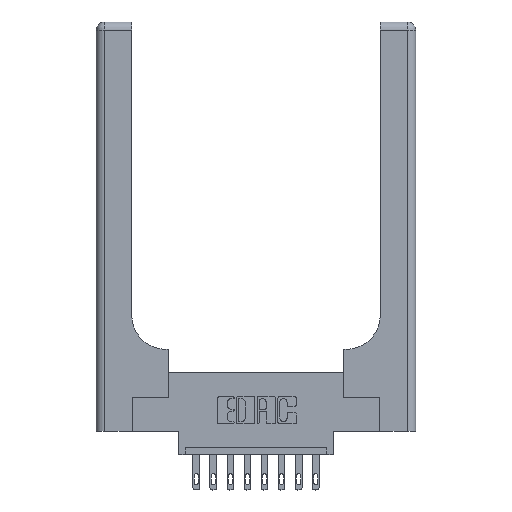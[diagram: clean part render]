
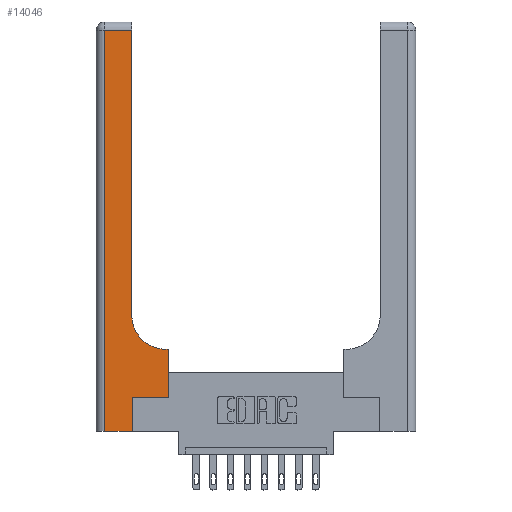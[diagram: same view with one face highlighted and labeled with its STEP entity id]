
A CAD part, top view. The second image highlights one B-rep face of the part: STEP entity #14046.
In plain terms, the highlighted planar face has unit normal (0, 0, 1).
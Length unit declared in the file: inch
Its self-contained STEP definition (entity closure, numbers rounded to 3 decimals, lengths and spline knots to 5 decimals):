
#158 = CARTESIAN_POINT ( 'NONE',  ( 0.265, 0., 0.37 ) ) ;
#459 = LINE ( 'NONE', #7547, #9441 ) ;
#603 = CARTESIAN_POINT ( 'NONE',  ( 0.26, 3., 0.37 ) ) ;
#756 = EDGE_LOOP ( 'NONE', ( #848, #13012, #11049, #14284, #3044, #6125, #1793, #9005, #6322 ) ) ;
#787 = CARTESIAN_POINT ( 'NONE',  ( 0.26, 2.94, 0.37 ) ) ;
#848 = ORIENTED_EDGE ( 'NONE', *, *, #12270, .T. ) ;
#910 = CARTESIAN_POINT ( 'NONE',  ( 0.26, 0.6, 0.37 ) ) ;
#918 = CARTESIAN_POINT ( 'NONE',  ( 0.528, 0.6, 0.37 ) ) ;
#1620 = LINE ( 'NONE', #603, #10219 ) ;
#1672 = DIRECTION ( 'NONE',  ( 0., -1., 0. ) ) ;
#1793 = ORIENTED_EDGE ( 'NONE', *, *, #2515, .T. ) ;
#2161 = VECTOR ( 'NONE', #14399, 39.37008 ) ;
#2469 = LINE ( 'NONE', #7157, #3348 ) ;
#2515 = EDGE_CURVE ( 'NONE', #13870, #5952, #8807, .T. ) ;
#3044 = ORIENTED_EDGE ( 'NONE', *, *, #3825, .T. ) ;
#3224 = CARTESIAN_POINT ( 'NONE',  ( 0.26, 0.85, 0.37 ) ) ;
#3348 = VECTOR ( 'NONE', #13458, 39.37008 ) ;
#3782 = VERTEX_POINT ( 'NONE', #4012 ) ;
#3825 = EDGE_CURVE ( 'NONE', #9197, #3782, #459, .T. ) ;
#3858 = DIRECTION ( 'NONE',  ( 0., 1., 0. ) ) ;
#4012 = CARTESIAN_POINT ( 'NONE',  ( 0.265, 0.25, 0.37 ) ) ;
#4062 = CARTESIAN_POINT ( 'NONE',  ( 0.06, 3., 0.37 ) ) ;
#4175 = CARTESIAN_POINT ( 'NONE',  ( 0.06, 2.94, 0.37 ) ) ;
#4379 = CARTESIAN_POINT ( 'NONE',  ( 0.51, 0.6, 0.37 ) ) ;
#4477 = DIRECTION ( 'NONE',  ( -1., 0., 0. ) ) ;
#4749 = VERTEX_POINT ( 'NONE', #4175 ) ;
#4796 = EDGE_CURVE ( 'NONE', #11384, #4749, #5330, .T. ) ;
#4879 = CARTESIAN_POINT ( 'NONE',  ( 0.265, 0.25, 0.37 ) ) ;
#5036 = LINE ( 'NONE', #4879, #2161 ) ;
#5330 = LINE ( 'NONE', #10004, #14877 ) ;
#5911 = CARTESIAN_POINT ( 'NONE',  ( 0.528, 0.25, 0.37 ) ) ;
#5952 = VERTEX_POINT ( 'NONE', #918 ) ;
#6125 = ORIENTED_EDGE ( 'NONE', *, *, #10378, .T. ) ;
#6128 = AXIS2_PLACEMENT_3D ( 'NONE', #6481, #12416, #11115 ) ;
#6322 = ORIENTED_EDGE ( 'NONE', *, *, #10534, .T. ) ;
#6481 = CARTESIAN_POINT ( 'NONE',  ( 0.51, 0.85, 0.37 ) ) ;
#6900 = VECTOR ( 'NONE', #1672, 39.37008 ) ;
#7157 = CARTESIAN_POINT ( 'NONE',  ( 0., 0., 0.37 ) ) ;
#7434 = CARTESIAN_POINT ( 'NONE',  ( 0., 3., 0.37 ) ) ;
#7547 = CARTESIAN_POINT ( 'NONE',  ( 0.265, 0., 0.37 ) ) ;
#7729 = VERTEX_POINT ( 'NONE', #4379 ) ;
#8346 = EDGE_CURVE ( 'NONE', #4749, #13665, #11228, .T. ) ;
#8807 = LINE ( 'NONE', #12158, #14511 ) ;
#9005 = ORIENTED_EDGE ( 'NONE', *, *, #12449, .T. ) ;
#9197 = VERTEX_POINT ( 'NONE', #158 ) ;
#9318 = VECTOR ( 'NONE', #4477, 39.37008 ) ;
#9441 = VECTOR ( 'NONE', #3858, 39.37008 ) ;
#9690 = DIRECTION ( 'NONE',  ( 0., 1., 0. ) ) ;
#9823 = DIRECTION ( 'NONE',  ( 0., 1., 0. ) ) ;
#9975 = CARTESIAN_POINT ( 'NONE',  ( 0.06, 0., 0.37 ) ) ;
#10004 = CARTESIAN_POINT ( 'NONE',  ( 0., 2.94, 0.37 ) ) ;
#10219 = VECTOR ( 'NONE', #9690, 39.37008 ) ;
#10378 = EDGE_CURVE ( 'NONE', #3782, #13870, #5036, .T. ) ;
#10525 = CIRCLE ( 'NONE', #6128, 0.25 ) ;
#10534 = EDGE_CURVE ( 'NONE', #7729, #15166, #10525, .T. ) ;
#11049 = ORIENTED_EDGE ( 'NONE', *, *, #8346, .T. ) ;
#11062 = DIRECTION ( 'NONE',  ( 0., 0., -1. ) ) ;
#11115 = DIRECTION ( 'NONE',  ( 1., 0., 0. ) ) ;
#11143 = DIRECTION ( 'NONE',  ( -1., 0., 0. ) ) ;
#11228 = LINE ( 'NONE', #4062, #6900 ) ;
#11384 = VERTEX_POINT ( 'NONE', #787 ) ;
#11720 = AXIS2_PLACEMENT_3D ( 'NONE', #7434, #11062, #11143 ) ;
#12064 = PLANE ( 'NONE',  #11720 ) ;
#12158 = CARTESIAN_POINT ( 'NONE',  ( 0.528, 0.25, 0.37 ) ) ;
#12270 = EDGE_CURVE ( 'NONE', #15166, #11384, #1620, .T. ) ;
#12416 = DIRECTION ( 'NONE',  ( 0., 0., -1. ) ) ;
#12449 = EDGE_CURVE ( 'NONE', #5952, #7729, #12706, .T. ) ;
#12706 = LINE ( 'NONE', #910, #9318 ) ;
#13012 = ORIENTED_EDGE ( 'NONE', *, *, #4796, .T. ) ;
#13458 = DIRECTION ( 'NONE',  ( 1., 0., 0. ) ) ;
#13576 = EDGE_CURVE ( 'NONE', #13665, #9197, #2469, .T. ) ;
#13665 = VERTEX_POINT ( 'NONE', #9975 ) ;
#13870 = VERTEX_POINT ( 'NONE', #5911 ) ;
#14046 = ADVANCED_FACE ( 'NONE', ( #14355 ), #12064, .F. ) ;
#14284 = ORIENTED_EDGE ( 'NONE', *, *, #13576, .T. ) ;
#14355 = FACE_OUTER_BOUND ( 'NONE', #756, .T. ) ;
#14399 = DIRECTION ( 'NONE',  ( 1., 0., 0. ) ) ;
#14511 = VECTOR ( 'NONE', #9823, 39.37008 ) ;
#14697 = DIRECTION ( 'NONE',  ( -1., 0., 0. ) ) ;
#14877 = VECTOR ( 'NONE', #14697, 39.37008 ) ;
#15166 = VERTEX_POINT ( 'NONE', #3224 ) ;
